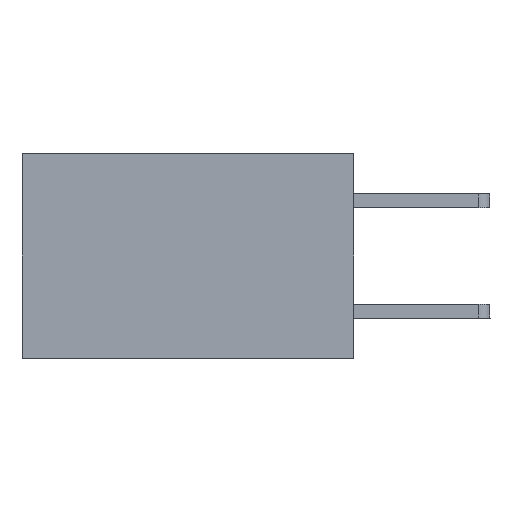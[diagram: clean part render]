
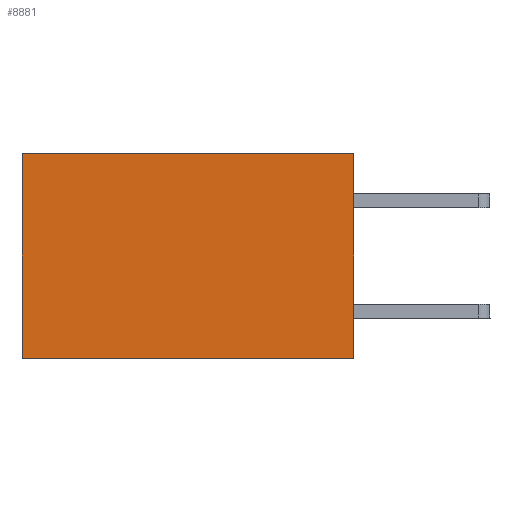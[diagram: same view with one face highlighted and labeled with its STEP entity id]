
A CAD part, left-side view. The second image highlights one B-rep face of the part: STEP entity #8881.
In plain terms, the highlighted planar face has unit normal (-1, 0, 0).
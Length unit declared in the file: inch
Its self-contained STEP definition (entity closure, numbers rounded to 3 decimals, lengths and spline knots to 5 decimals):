
#38 = VERTEX_POINT ( 'NONE', #5001 ) ;
#282 = AXIS2_PLACEMENT_3D ( 'NONE', #3122, #4301, #13279 ) ;
#654 = DIRECTION ( 'NONE',  ( 0., 0., -1. ) ) ;
#1089 = PLANE ( 'NONE',  #282 ) ;
#1557 = EDGE_LOOP ( 'NONE', ( #8380, #6286, #7728, #9433 ) ) ;
#1763 = LINE ( 'NONE', #9715, #6862 ) ;
#1829 = CARTESIAN_POINT ( 'NONE',  ( 0.2875, 0., 0. ) ) ;
#2252 = EDGE_CURVE ( 'NONE', #38, #5394, #5119, .T. ) ;
#3122 = CARTESIAN_POINT ( 'NONE',  ( 0.2875, 0., 0. ) ) ;
#3583 = VERTEX_POINT ( 'NONE', #9396 ) ;
#3877 = DIRECTION ( 'NONE',  ( 0., 0., -1. ) ) ;
#4301 = DIRECTION ( 'NONE',  ( 1., 0., 0. ) ) ;
#4341 = DIRECTION ( 'NONE',  ( 0., 1., 0. ) ) ;
#5001 = CARTESIAN_POINT ( 'NONE',  ( 0.2875, 0., 0. ) ) ;
#5119 = LINE ( 'NONE', #1829, #12946 ) ;
#5394 = VERTEX_POINT ( 'NONE', #14203 ) ;
#5471 = FACE_OUTER_BOUND ( 'NONE', #1557, .T. ) ;
#6027 = EDGE_CURVE ( 'NONE', #38, #10612, #14399, .T. ) ;
#6286 = ORIENTED_EDGE ( 'NONE', *, *, #11126, .F. ) ;
#6862 = VECTOR ( 'NONE', #3877, 39.37008 ) ;
#7458 = VECTOR ( 'NONE', #654, 39.37008 ) ;
#7728 = ORIENTED_EDGE ( 'NONE', *, *, #6027, .F. ) ;
#7769 = CARTESIAN_POINT ( 'NONE',  ( 0.2875, 0., -0.37 ) ) ;
#8380 = ORIENTED_EDGE ( 'NONE', *, *, #11372, .T. ) ;
#8881 = ADVANCED_FACE ( 'NONE', ( #5471 ), #1089, .F. ) ;
#9396 = CARTESIAN_POINT ( 'NONE',  ( 0.2875, 0.6, -0.37 ) ) ;
#9417 = DIRECTION ( 'NONE',  ( 0., 1., 0. ) ) ;
#9433 = ORIENTED_EDGE ( 'NONE', *, *, #2252, .T. ) ;
#9715 = CARTESIAN_POINT ( 'NONE',  ( 0.2875, 0.6, 0. ) ) ;
#10612 = VERTEX_POINT ( 'NONE', #14144 ) ;
#10984 = LINE ( 'NONE', #7769, #11760 ) ;
#11126 = EDGE_CURVE ( 'NONE', #10612, #3583, #10984, .T. ) ;
#11372 = EDGE_CURVE ( 'NONE', #5394, #3583, #1763, .T. ) ;
#11760 = VECTOR ( 'NONE', #4341, 39.37008 ) ;
#12946 = VECTOR ( 'NONE', #9417, 39.37008 ) ;
#13279 = DIRECTION ( 'NONE',  ( 0., 0., -1. ) ) ;
#13462 = CARTESIAN_POINT ( 'NONE',  ( 0.2875, 0., 0. ) ) ;
#14144 = CARTESIAN_POINT ( 'NONE',  ( 0.2875, 0., -0.37 ) ) ;
#14203 = CARTESIAN_POINT ( 'NONE',  ( 0.2875, 0.6, 0. ) ) ;
#14399 = LINE ( 'NONE', #13462, #7458 ) ;
